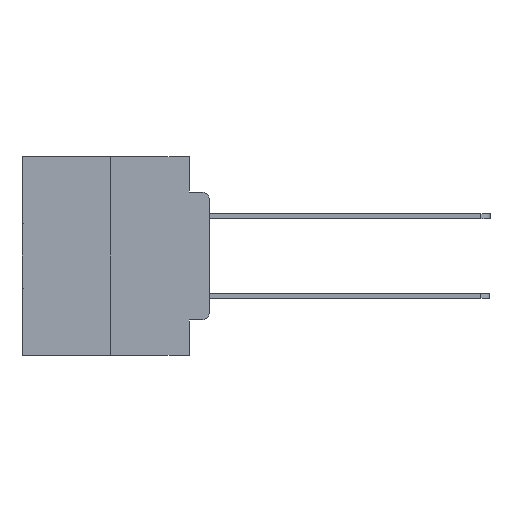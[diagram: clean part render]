
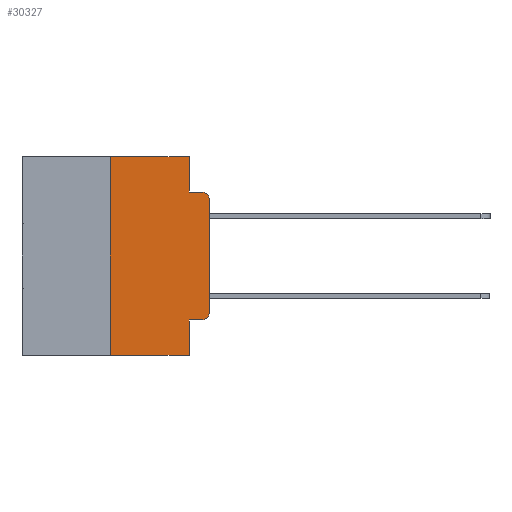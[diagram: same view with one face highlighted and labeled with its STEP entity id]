
A CAD part, left-side view. The second image highlights one B-rep face of the part: STEP entity #30327.
In plain terms, the highlighted planar face has unit normal (-1, 0, 0).
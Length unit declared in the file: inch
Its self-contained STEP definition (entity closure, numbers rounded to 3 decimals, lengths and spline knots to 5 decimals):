
#1487 = CARTESIAN_POINT ( 'NONE',  ( 0., 0.051, 0. ) ) ;
#3406 = VERTEX_POINT ( 'NONE', #1487 ) ;
#3975 = CARTESIAN_POINT ( 'NONE',  ( 0., 0.25, -0.5 ) ) ;
#4296 = DIRECTION ( 'NONE',  ( 0., 0., -1. ) ) ;
#4662 = ORIENTED_EDGE ( 'NONE', *, *, #15970, .T. ) ;
#5201 = CARTESIAN_POINT ( 'NONE',  ( 0., 0.25, 0. ) ) ;
#5262 = ORIENTED_EDGE ( 'NONE', *, *, #7564, .F. ) ;
#5457 = ORIENTED_EDGE ( 'NONE', *, *, #12427, .T. ) ;
#6262 = CARTESIAN_POINT ( 'NONE',  ( 0., 0.02, -0.3915 ) ) ;
#6307 = DIRECTION ( 'NONE',  ( 0., -1., 0. ) ) ;
#6688 = CIRCLE ( 'NONE', #25968, 0.02 ) ;
#6882 = VECTOR ( 'NONE', #23808, 39.37008 ) ;
#7459 = VERTEX_POINT ( 'NONE', #26385 ) ;
#7555 = DIRECTION ( 'NONE',  ( 0., 0., 1. ) ) ;
#7564 = EDGE_CURVE ( 'NONE', #8308, #3406, #16799, .T. ) ;
#7866 = CARTESIAN_POINT ( 'NONE',  ( 0., 0., -0.3915 ) ) ;
#8308 = VERTEX_POINT ( 'NONE', #5201 ) ;
#8339 = ORIENTED_EDGE ( 'NONE', *, *, #22442, .F. ) ;
#8537 = LINE ( 'NONE', #22056, #15015 ) ;
#8565 = CARTESIAN_POINT ( 'NONE',  ( 0., 0.051, -0.4115 ) ) ;
#8608 = ORIENTED_EDGE ( 'NONE', *, *, #21553, .T. ) ;
#8782 = DIRECTION ( 'NONE',  ( 0., 0., -1. ) ) ;
#8837 = CARTESIAN_POINT ( 'NONE',  ( 0., 0.473, -0.5 ) ) ;
#9219 = CARTESIAN_POINT ( 'NONE',  ( 0., 0.051, -0.0885 ) ) ;
#9325 = VECTOR ( 'NONE', #9446, 39.37008 ) ;
#9446 = DIRECTION ( 'NONE',  ( 0., 0., -1. ) ) ;
#9572 = DIRECTION ( 'NONE',  ( 0., -1., 0. ) ) ;
#10145 = ORIENTED_EDGE ( 'NONE', *, *, #31136, .F. ) ;
#10339 = ORIENTED_EDGE ( 'NONE', *, *, #24175, .T. ) ;
#10702 = ORIENTED_EDGE ( 'NONE', *, *, #29380, .F. ) ;
#10905 = CARTESIAN_POINT ( 'NONE',  ( 0., 0.25, 0. ) ) ;
#11022 = VERTEX_POINT ( 'NONE', #3975 ) ;
#11330 = CARTESIAN_POINT ( 'NONE',  ( 0., 0.02, -0.4115 ) ) ;
#11442 = VERTEX_POINT ( 'NONE', #27454 ) ;
#11992 = CARTESIAN_POINT ( 'NONE',  ( 0., 0.051, -0.0885 ) ) ;
#12002 = CARTESIAN_POINT ( 'NONE',  ( 0., 0.473, 0. ) ) ;
#12258 = CARTESIAN_POINT ( 'NONE',  ( 0., 0.473, 0. ) ) ;
#12373 = DIRECTION ( 'NONE',  ( -1., 0., 0. ) ) ;
#12427 = EDGE_CURVE ( 'NONE', #26896, #29810, #8537, .T. ) ;
#12635 = LINE ( 'NONE', #16568, #6882 ) ;
#12671 = CARTESIAN_POINT ( 'NONE',  ( 0., 0., -0.1085 ) ) ;
#14058 = LINE ( 'NONE', #10905, #19722 ) ;
#14126 = CARTESIAN_POINT ( 'NONE',  ( 0., 0.051, 0. ) ) ;
#14462 = DIRECTION ( 'NONE',  ( 1., 0., 0. ) ) ;
#15015 = VECTOR ( 'NONE', #7555, 39.37008 ) ;
#15684 = VECTOR ( 'NONE', #4296, 39.37008 ) ;
#15755 = EDGE_LOOP ( 'NONE', ( #5457, #4662, #10145, #8339, #5262, #10702, #10339, #23634, #21849, #8608 ) ) ;
#15781 = VERTEX_POINT ( 'NONE', #9219 ) ;
#15970 = EDGE_CURVE ( 'NONE', #29810, #11442, #6688, .T. ) ;
#16568 = CARTESIAN_POINT ( 'NONE',  ( 0., 0.051, -0.4115 ) ) ;
#16755 = LINE ( 'NONE', #8837, #22373 ) ;
#16799 = LINE ( 'NONE', #12258, #28800 ) ;
#17804 = AXIS2_PLACEMENT_3D ( 'NONE', #6262, #23243, #8782 ) ;
#18838 = EDGE_CURVE ( 'NONE', #25892, #23037, #12635, .T. ) ;
#19722 = VECTOR ( 'NONE', #27759, 39.37008 ) ;
#20413 = FACE_OUTER_BOUND ( 'NONE', #15755, .T. ) ;
#21127 = EDGE_CURVE ( 'NONE', #25892, #7459, #21437, .T. ) ;
#21437 = LINE ( 'NONE', #23899, #9325 ) ;
#21553 = EDGE_CURVE ( 'NONE', #23037, #26896, #29255, .T. ) ;
#21849 = ORIENTED_EDGE ( 'NONE', *, *, #18838, .T. ) ;
#22056 = CARTESIAN_POINT ( 'NONE',  ( 0., 0., 0. ) ) ;
#22078 = LINE ( 'NONE', #14126, #15684 ) ;
#22373 = VECTOR ( 'NONE', #6307, 39.37008 ) ;
#22442 = EDGE_CURVE ( 'NONE', #3406, #15781, #22078, .T. ) ;
#23037 = VERTEX_POINT ( 'NONE', #11330 ) ;
#23243 = DIRECTION ( 'NONE',  ( -1., 0., 0. ) ) ;
#23634 = ORIENTED_EDGE ( 'NONE', *, *, #21127, .F. ) ;
#23808 = DIRECTION ( 'NONE',  ( 0., -1., 0. ) ) ;
#23899 = CARTESIAN_POINT ( 'NONE',  ( 0., 0.051, 0. ) ) ;
#24034 = AXIS2_PLACEMENT_3D ( 'NONE', #12002, #14462, #31243 ) ;
#24175 = EDGE_CURVE ( 'NONE', #11022, #7459, #16755, .T. ) ;
#25892 = VERTEX_POINT ( 'NONE', #8565 ) ;
#25968 = AXIS2_PLACEMENT_3D ( 'NONE', #26815, #12373, #29207 ) ;
#26385 = CARTESIAN_POINT ( 'NONE',  ( 0., 0.051, -0.5 ) ) ;
#26453 = PLANE ( 'NONE',  #24034 ) ;
#26745 = VECTOR ( 'NONE', #9572, 39.37008 ) ;
#26815 = CARTESIAN_POINT ( 'NONE',  ( 0., 0.02, -0.1085 ) ) ;
#26896 = VERTEX_POINT ( 'NONE', #7866 ) ;
#27454 = CARTESIAN_POINT ( 'NONE',  ( 0., 0.02, -0.0885 ) ) ;
#27483 = LINE ( 'NONE', #11992, #26745 ) ;
#27759 = DIRECTION ( 'NONE',  ( 0., 0., 1. ) ) ;
#28800 = VECTOR ( 'NONE', #28881, 39.37008 ) ;
#28881 = DIRECTION ( 'NONE',  ( 0., -1., 0. ) ) ;
#29207 = DIRECTION ( 'NONE',  ( 0., 0., -1. ) ) ;
#29255 = CIRCLE ( 'NONE', #17804, 0.02 ) ;
#29380 = EDGE_CURVE ( 'NONE', #11022, #8308, #14058, .T. ) ;
#29810 = VERTEX_POINT ( 'NONE', #12671 ) ;
#30327 = ADVANCED_FACE ( 'NONE', ( #20413 ), #26453, .F. ) ;
#31136 = EDGE_CURVE ( 'NONE', #15781, #11442, #27483, .T. ) ;
#31243 = DIRECTION ( 'NONE',  ( 0., 0., -1. ) ) ;
